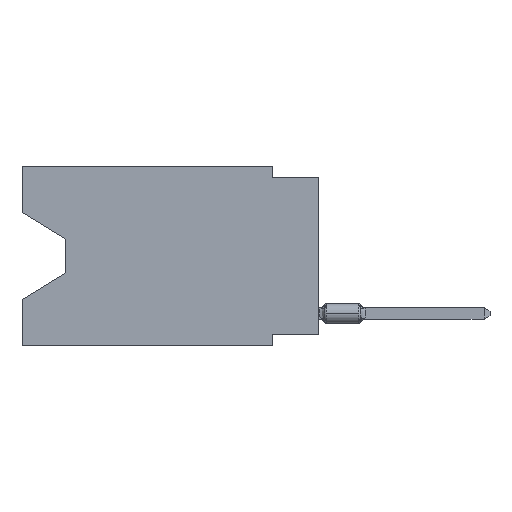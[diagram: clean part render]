
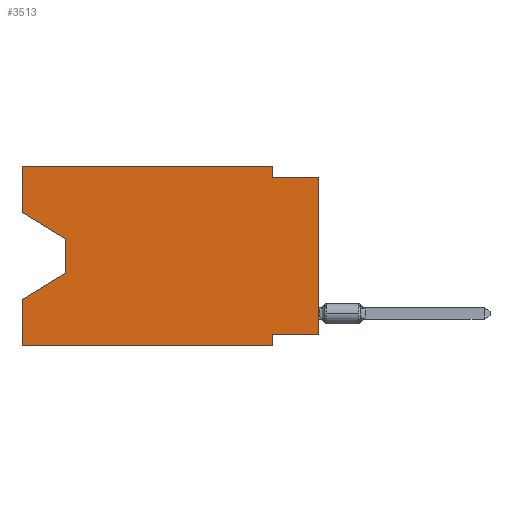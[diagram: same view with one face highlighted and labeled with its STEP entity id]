
A CAD part, left-side view. The second image highlights one B-rep face of the part: STEP entity #3513.
In plain terms, the highlighted planar face has unit normal (-1, 0, 0).
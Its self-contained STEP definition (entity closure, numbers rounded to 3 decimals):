
#27 = LINE ( 'NONE', #6531, #12200 ) ;
#70 = VECTOR ( 'NONE', #6207, 1000. ) ;
#157 = CARTESIAN_POINT ( 'NONE',  ( 0., 2.54, 0. ) ) ;
#171 = DIRECTION ( 'NONE',  ( 0., 0., -1. ) ) ;
#424 = EDGE_CURVE ( 'NONE', #4499, #2949, #11878, .T. ) ;
#1007 = EDGE_CURVE ( 'NONE', #4070, #2238, #14016, .T. ) ;
#1094 = DIRECTION ( 'NONE',  ( 0., 0., 1. ) ) ;
#1150 = VECTOR ( 'NONE', #5011, 1000. ) ;
#1204 = VECTOR ( 'NONE', #3363, 1000. ) ;
#1307 = LINE ( 'NONE', #11852, #3095 ) ;
#1324 = CARTESIAN_POINT ( 'NONE',  ( 0., 13.97, -4.013 ) ) ;
#1423 = CARTESIAN_POINT ( 'NONE',  ( 0., 16.383, 0. ) ) ;
#1531 = CARTESIAN_POINT ( 'NONE',  ( 0., 0., -9.271 ) ) ;
#1572 = PLANE ( 'NONE',  #2761 ) ;
#1573 = EDGE_CURVE ( 'NONE', #13220, #9070, #1307, .T. ) ;
#1638 = ORIENTED_EDGE ( 'NONE', *, *, #7740, .F. ) ;
#2087 = CARTESIAN_POINT ( 'NONE',  ( 0., 2.54, -9.271 ) ) ;
#2238 = VERTEX_POINT ( 'NONE', #13864 ) ;
#2312 = VECTOR ( 'NONE', #3470, 1000. ) ;
#2584 = ORIENTED_EDGE ( 'NONE', *, *, #4172, .T. ) ;
#2731 = LINE ( 'NONE', #157, #2312 ) ;
#2761 = AXIS2_PLACEMENT_3D ( 'NONE', #1423, #2910, #171 ) ;
#2839 = EDGE_CURVE ( 'NONE', #4499, #13756, #13586, .T. ) ;
#2910 = DIRECTION ( 'NONE',  ( 1., 0., 0. ) ) ;
#2949 = VERTEX_POINT ( 'NONE', #6900 ) ;
#2967 = VECTOR ( 'NONE', #4267, 1000. ) ;
#2991 = VERTEX_POINT ( 'NONE', #10441 ) ;
#3095 = VECTOR ( 'NONE', #10994, 1000. ) ;
#3124 = ORIENTED_EDGE ( 'NONE', *, *, #9592, .T. ) ;
#3354 = EDGE_CURVE ( 'NONE', #2949, #13662, #5610, .T. ) ;
#3363 = DIRECTION ( 'NONE',  ( 0., -1., 0. ) ) ;
#3470 = DIRECTION ( 'NONE',  ( 0., 0., -1. ) ) ;
#3513 = ADVANCED_FACE ( 'NONE', ( #13455 ), #1572, .F. ) ;
#3917 = CARTESIAN_POINT ( 'NONE',  ( 0., 16.383, -2.546 ) ) ;
#4070 = VERTEX_POINT ( 'NONE', #6519 ) ;
#4172 = EDGE_CURVE ( 'NONE', #13733, #7888, #9354, .T. ) ;
#4193 = CARTESIAN_POINT ( 'NONE',  ( 0., 2.54, 0. ) ) ;
#4260 = DIRECTION ( 'NONE',  ( 0., -1., 0. ) ) ;
#4267 = DIRECTION ( 'NONE',  ( 0., 0., 1. ) ) ;
#4301 = VECTOR ( 'NONE', #12679, 1000. ) ;
#4499 = VERTEX_POINT ( 'NONE', #5473 ) ;
#4535 = VECTOR ( 'NONE', #9596, 1000. ) ;
#4732 = EDGE_CURVE ( 'NONE', #13733, #2991, #15049, .T. ) ;
#4770 = LINE ( 'NONE', #1324, #4535 ) ;
#4807 = ORIENTED_EDGE ( 'NONE', *, *, #11579, .T. ) ;
#5011 = DIRECTION ( 'NONE',  ( 0., -0.855, -0.519 ) ) ;
#5473 = CARTESIAN_POINT ( 'NONE',  ( 0., 16.383, -2.546 ) ) ;
#5573 = ORIENTED_EDGE ( 'NONE', *, *, #4732, .F. ) ;
#5610 = LINE ( 'NONE', #7820, #13069 ) ;
#5841 = EDGE_CURVE ( 'NONE', #13220, #2238, #7397, .T. ) ;
#5897 = CARTESIAN_POINT ( 'NONE',  ( 0., 16.383, 0. ) ) ;
#6207 = DIRECTION ( 'NONE',  ( 0., 0., 1. ) ) ;
#6519 = CARTESIAN_POINT ( 'NONE',  ( 0., 2.54, -0.635 ) ) ;
#6531 = CARTESIAN_POINT ( 'NONE',  ( 0., 2.54, -9.906 ) ) ;
#6638 = CARTESIAN_POINT ( 'NONE',  ( 0., 0., -0.635 ) ) ;
#6900 = CARTESIAN_POINT ( 'NONE',  ( 0., 16.383, 0. ) ) ;
#7397 = LINE ( 'NONE', #12178, #70 ) ;
#7740 = EDGE_CURVE ( 'NONE', #9070, #7888, #27, .T. ) ;
#7820 = CARTESIAN_POINT ( 'NONE',  ( 0., 16.383, 0. ) ) ;
#7888 = VERTEX_POINT ( 'NONE', #9143 ) ;
#8766 = CARTESIAN_POINT ( 'NONE',  ( 0., 16.383, -9.906 ) ) ;
#9070 = VERTEX_POINT ( 'NONE', #2087 ) ;
#9143 = CARTESIAN_POINT ( 'NONE',  ( 0., 2.54, -9.906 ) ) ;
#9354 = LINE ( 'NONE', #14144, #1204 ) ;
#9592 = EDGE_CURVE ( 'NONE', #14688, #2991, #13533, .T. ) ;
#9596 = DIRECTION ( 'NONE',  ( 0., 0., -1. ) ) ;
#9712 = VECTOR ( 'NONE', #1094, 1000. ) ;
#10108 = VECTOR ( 'NONE', #13384, 1000. ) ;
#10441 = CARTESIAN_POINT ( 'NONE',  ( 0., 16.383, -7.36 ) ) ;
#10994 = DIRECTION ( 'NONE',  ( 0., 1., 0. ) ) ;
#11034 = CARTESIAN_POINT ( 'NONE',  ( 0., 13.97, -5.893 ) ) ;
#11520 = CARTESIAN_POINT ( 'NONE',  ( 0., 16.383, 0. ) ) ;
#11579 = EDGE_CURVE ( 'NONE', #13756, #14688, #4770, .T. ) ;
#11852 = CARTESIAN_POINT ( 'NONE',  ( 0., 0., -9.271 ) ) ;
#11878 = LINE ( 'NONE', #5897, #9712 ) ;
#11999 = CARTESIAN_POINT ( 'NONE',  ( 0., 13.97, -5.893 ) ) ;
#12061 = DIRECTION ( 'NONE',  ( 0., 0., -1. ) ) ;
#12178 = CARTESIAN_POINT ( 'NONE',  ( 0., 0., 0. ) ) ;
#12200 = VECTOR ( 'NONE', #12061, 1000. ) ;
#12666 = ORIENTED_EDGE ( 'NONE', *, *, #3354, .F. ) ;
#12679 = DIRECTION ( 'NONE',  ( 0., -1., 0. ) ) ;
#12784 = ORIENTED_EDGE ( 'NONE', *, *, #13981, .F. ) ;
#12888 = ORIENTED_EDGE ( 'NONE', *, *, #424, .F. ) ;
#13069 = VECTOR ( 'NONE', #4260, 1000. ) ;
#13220 = VERTEX_POINT ( 'NONE', #1531 ) ;
#13245 = ORIENTED_EDGE ( 'NONE', *, *, #1573, .F. ) ;
#13257 = ORIENTED_EDGE ( 'NONE', *, *, #1007, .F. ) ;
#13384 = DIRECTION ( 'NONE',  ( 0., 0.855, -0.519 ) ) ;
#13455 = FACE_OUTER_BOUND ( 'NONE', #15135, .T. ) ;
#13533 = LINE ( 'NONE', #11034, #10108 ) ;
#13586 = LINE ( 'NONE', #3917, #1150 ) ;
#13635 = CARTESIAN_POINT ( 'NONE',  ( 0., 13.97, -4.013 ) ) ;
#13662 = VERTEX_POINT ( 'NONE', #4193 ) ;
#13733 = VERTEX_POINT ( 'NONE', #8766 ) ;
#13756 = VERTEX_POINT ( 'NONE', #13635 ) ;
#13864 = CARTESIAN_POINT ( 'NONE',  ( 0., 0., -0.635 ) ) ;
#13981 = EDGE_CURVE ( 'NONE', #13662, #4070, #2731, .T. ) ;
#14016 = LINE ( 'NONE', #6638, #4301 ) ;
#14144 = CARTESIAN_POINT ( 'NONE',  ( 0., 16.383, -9.906 ) ) ;
#14688 = VERTEX_POINT ( 'NONE', #11999 ) ;
#14759 = ORIENTED_EDGE ( 'NONE', *, *, #2839, .T. ) ;
#14916 = ORIENTED_EDGE ( 'NONE', *, *, #5841, .T. ) ;
#15049 = LINE ( 'NONE', #11520, #2967 ) ;
#15135 = EDGE_LOOP ( 'NONE', ( #14759, #4807, #3124, #5573, #2584, #1638, #13245, #14916, #13257, #12784, #12666, #12888 ) ) ;
